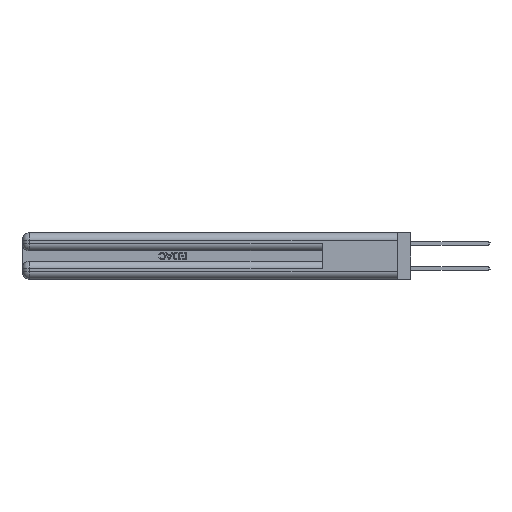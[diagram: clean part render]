
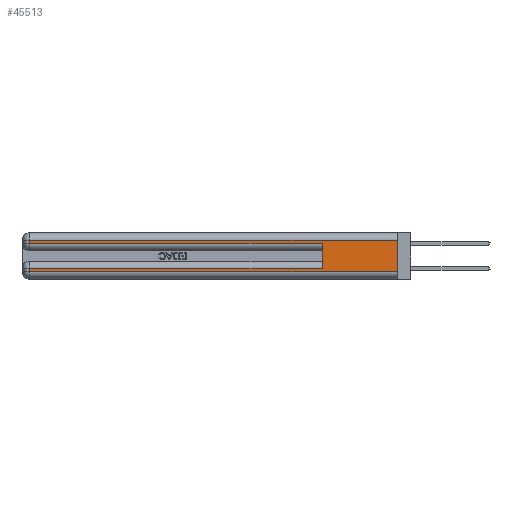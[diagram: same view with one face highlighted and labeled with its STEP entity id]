
A CAD part, left-side view. The second image highlights one B-rep face of the part: STEP entity #45513.
In plain terms, the highlighted planar face has unit normal (-1, 0, 0).
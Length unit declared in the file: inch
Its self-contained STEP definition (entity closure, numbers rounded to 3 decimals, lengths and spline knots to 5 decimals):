
#812 = CARTESIAN_POINT ( 'NONE',  ( 0., 0., 0.31 ) ) ;
#1231 = CARTESIAN_POINT ( 'NONE',  ( 0., 0.6, 0.085 ) ) ;
#1295 = VERTEX_POINT ( 'NONE', #25812 ) ;
#2639 = CARTESIAN_POINT ( 'NONE',  ( 0., 2.94, 0.085 ) ) ;
#2744 = CARTESIAN_POINT ( 'NONE',  ( 0., 2.94, 0.31 ) ) ;
#3227 = DIRECTION ( 'NONE',  ( 0., 0., -1. ) ) ;
#3477 = CARTESIAN_POINT ( 'NONE',  ( 0., 0., 0.06 ) ) ;
#3997 = DIRECTION ( 'NONE',  ( 0., -1., 0. ) ) ;
#4327 = ORIENTED_EDGE ( 'NONE', *, *, #45218, .F. ) ;
#4520 = DIRECTION ( 'NONE',  ( 0., 1., 0. ) ) ;
#4705 = VERTEX_POINT ( 'NONE', #2744 ) ;
#5279 = DIRECTION ( 'NONE',  ( 0., 0., -1. ) ) ;
#6344 = VECTOR ( 'NONE', #25578, 39.37008 ) ;
#7501 = CARTESIAN_POINT ( 'NONE',  ( 0., 2.94, 0.37 ) ) ;
#7701 = ORIENTED_EDGE ( 'NONE', *, *, #27015, .T. ) ;
#7734 = VECTOR ( 'NONE', #9327, 39.37008 ) ;
#8162 = ORIENTED_EDGE ( 'NONE', *, *, #46864, .F. ) ;
#8222 = LINE ( 'NONE', #19982, #37386 ) ;
#9207 = CARTESIAN_POINT ( 'NONE',  ( 0., 0., 0.285 ) ) ;
#9327 = DIRECTION ( 'NONE',  ( 0., 1., 0. ) ) ;
#10073 = ORIENTED_EDGE ( 'NONE', *, *, #42061, .T. ) ;
#10358 = CARTESIAN_POINT ( 'NONE',  ( 0., 0., 0.37 ) ) ;
#12927 = VERTEX_POINT ( 'NONE', #45421 ) ;
#13014 = CARTESIAN_POINT ( 'NONE',  ( 0., 0.6, 0.285 ) ) ;
#13089 = DIRECTION ( 'NONE',  ( 1., 0., 0. ) ) ;
#13643 = EDGE_CURVE ( 'NONE', #1295, #12927, #50114, .T. ) ;
#15535 = VERTEX_POINT ( 'NONE', #2639 ) ;
#16243 = VERTEX_POINT ( 'NONE', #812 ) ;
#16516 = ORIENTED_EDGE ( 'NONE', *, *, #20805, .T. ) ;
#17500 = EDGE_LOOP ( 'NONE', ( #8162, #16516, #49548, #41791, #4327, #10073, #7701, #44069 ) ) ;
#19374 = CARTESIAN_POINT ( 'NONE',  ( 0., 0.6, 0.145 ) ) ;
#19982 = CARTESIAN_POINT ( 'NONE',  ( 0., 0., 0.31 ) ) ;
#20805 = EDGE_CURVE ( 'NONE', #16243, #4705, #8222, .T. ) ;
#21313 = AXIS2_PLACEMENT_3D ( 'NONE', #37171, #13089, #5279 ) ;
#22320 = LINE ( 'NONE', #19374, #23576 ) ;
#23394 = DIRECTION ( 'NONE',  ( 0., 0., 1. ) ) ;
#23576 = VECTOR ( 'NONE', #23394, 39.37008 ) ;
#23668 = VECTOR ( 'NONE', #38541, 39.37008 ) ;
#25192 = LINE ( 'NONE', #35848, #7734 ) ;
#25578 = DIRECTION ( 'NONE',  ( 0., -1., 0. ) ) ;
#25812 = CARTESIAN_POINT ( 'NONE',  ( 0., 2.94, 0.06 ) ) ;
#27015 = EDGE_CURVE ( 'NONE', #15535, #1295, #42213, .T. ) ;
#28469 = LINE ( 'NONE', #10358, #43283 ) ;
#29839 = VECTOR ( 'NONE', #50191, 39.37008 ) ;
#29952 = LINE ( 'NONE', #9207, #6344 ) ;
#30077 = VERTEX_POINT ( 'NONE', #1231 ) ;
#32592 = CARTESIAN_POINT ( 'NONE',  ( 0., 2.94, 0.285 ) ) ;
#34484 = CARTESIAN_POINT ( 'NONE',  ( 0., 2.94, 0.37 ) ) ;
#35848 = CARTESIAN_POINT ( 'NONE',  ( 0., 0., 0.085 ) ) ;
#36764 = EDGE_CURVE ( 'NONE', #4705, #43969, #42218, .T. ) ;
#37171 = CARTESIAN_POINT ( 'NONE',  ( 0., 0., 0.37 ) ) ;
#37386 = VECTOR ( 'NONE', #4520, 39.37008 ) ;
#38541 = DIRECTION ( 'NONE',  ( 0., 0., -1. ) ) ;
#39623 = FACE_OUTER_BOUND ( 'NONE', #17500, .T. ) ;
#40649 = PLANE ( 'NONE',  #21313 ) ;
#41019 = VERTEX_POINT ( 'NONE', #13014 ) ;
#41791 = ORIENTED_EDGE ( 'NONE', *, *, #50766, .T. ) ;
#42061 = EDGE_CURVE ( 'NONE', #30077, #15535, #25192, .T. ) ;
#42213 = LINE ( 'NONE', #34484, #29839 ) ;
#42218 = LINE ( 'NONE', #7501, #23668 ) ;
#43283 = VECTOR ( 'NONE', #3227, 39.37008 ) ;
#43969 = VERTEX_POINT ( 'NONE', #32592 ) ;
#44069 = ORIENTED_EDGE ( 'NONE', *, *, #13643, .T. ) ;
#45218 = EDGE_CURVE ( 'NONE', #30077, #41019, #22320, .T. ) ;
#45421 = CARTESIAN_POINT ( 'NONE',  ( 0., 0., 0.06 ) ) ;
#45513 = ADVANCED_FACE ( 'NONE', ( #39623 ), #40649, .F. ) ;
#46864 = EDGE_CURVE ( 'NONE', #16243, #12927, #28469, .T. ) ;
#48904 = VECTOR ( 'NONE', #3997, 39.37008 ) ;
#49548 = ORIENTED_EDGE ( 'NONE', *, *, #36764, .T. ) ;
#50114 = LINE ( 'NONE', #3477, #48904 ) ;
#50191 = DIRECTION ( 'NONE',  ( 0., 0., -1. ) ) ;
#50766 = EDGE_CURVE ( 'NONE', #43969, #41019, #29952, .T. ) ;
